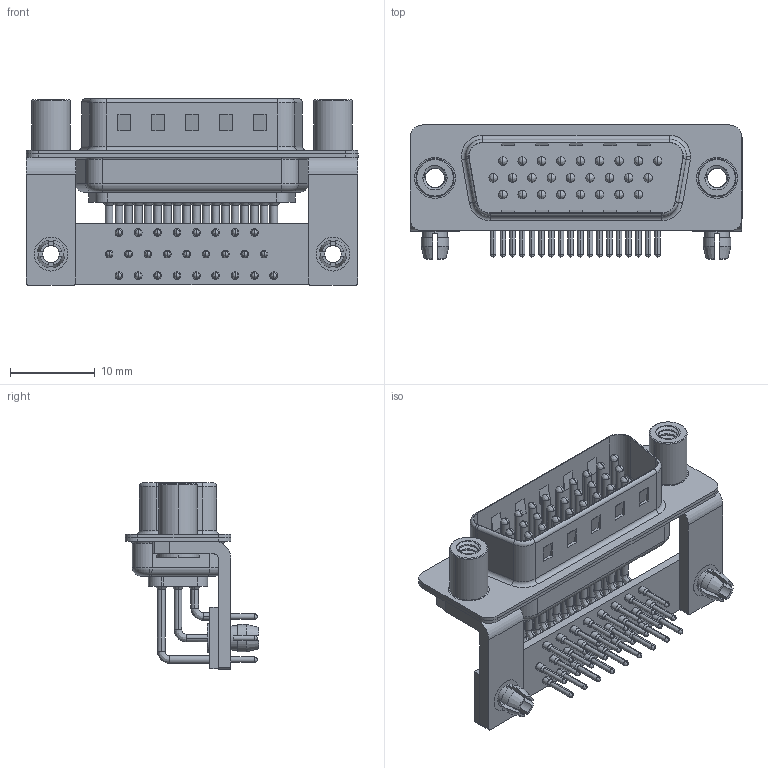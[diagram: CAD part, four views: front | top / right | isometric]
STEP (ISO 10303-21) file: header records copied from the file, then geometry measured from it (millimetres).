
FILE_DESCRIPTION (( 'STEP AP203' ), '1' );
FILE_NAME ('633-M26-363-WN5.STEP', '2018-09-27T23:20:27', ( '' ), ( '' ), 'SwSTEP 2.0', 'SolidWorks 2016', '' );
FILE_SCHEMA (( 'CONFIG_CONTROL_DESIGN' ));
Length unit declared in the file: millimetre
Products named in the file (11): 633-M26-363-WN5; 633M Shell Rear_26 Contacts; 633M Contact Row 1; 633M Contact Row 2; 633M Contact Row 3; 633M Stabilizer Bracket; 633M 4-40 Threaded Standoff; 633M Stabilizer Board_26 Contacts; 633M Housing_26 Contacts; 633M Board Lock; 633M Shell Front_26 Contacts
Assembly tree (36 placements, depth 2):
  633-M26-363-WN5
    633M Housing_26 Contacts
    633M Shell Front_26 Contacts
    633M Shell Rear_26 Contacts
    633M Contact Row 1  x9
    633M Contact Row 2  x9
    633M Contact Row 3  x8
    633M Stabilizer Bracket  x2
    633M 4-40 Threaded Standoff  x2
    633M Stabilizer Board_26 Contacts
    633M Board Lock  x2
Bounding box: 39.2 x 15.8 x 22 mm (x, y, z)
Volume: 2794.1 mm3; surface area: 8558.1 mm2
Topology: 36 solids, 36 shells, 3444 faces, 9605 edges, 6250 vertices
Faces by surface type: plane 1879, cylinder 1217, bspline 162, cone 130, torus 56
Entity records: 34304 total; most frequent: CARTESIAN_POINT 7475, DIRECTION 5445, ORIENTED_EDGE 5070, EDGE_CURVE 2535, AXIS2_PLACEMENT_3D 2007, VERTEX_POINT 1651, VECTOR 1431, LINE 1431
